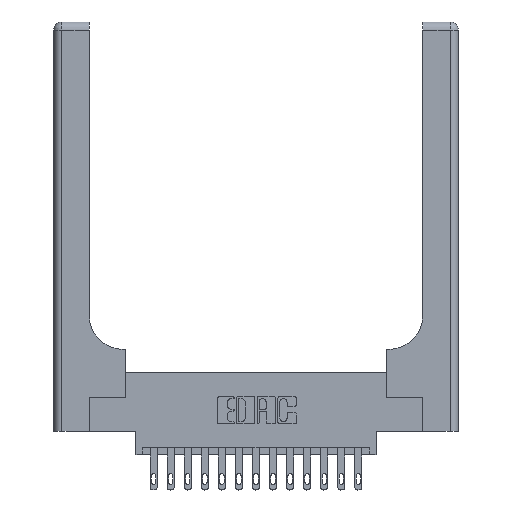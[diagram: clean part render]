
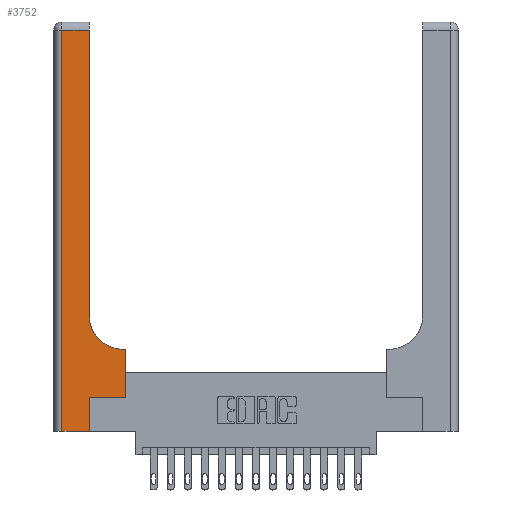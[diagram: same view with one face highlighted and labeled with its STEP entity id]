
A CAD part, top view. The second image highlights one B-rep face of the part: STEP entity #3752.
In plain terms, the highlighted planar face has unit normal (0, 0, 1).
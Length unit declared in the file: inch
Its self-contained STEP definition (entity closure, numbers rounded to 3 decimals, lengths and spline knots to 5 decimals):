
#110 = VECTOR ( 'NONE', #6248, 39.37008 ) ;
#417 = DIRECTION ( 'NONE',  ( -1., 0., 0. ) ) ;
#496 = DIRECTION ( 'NONE',  ( 0., 0., -1. ) ) ;
#1098 = VECTOR ( 'NONE', #417, 39.37008 ) ;
#1609 = VECTOR ( 'NONE', #12902, 39.37008 ) ;
#1746 = CARTESIAN_POINT ( 'NONE',  ( 0.528, 0.25, 0.37 ) ) ;
#1810 = ORIENTED_EDGE ( 'NONE', *, *, #6879, .T. ) ;
#2056 = ORIENTED_EDGE ( 'NONE', *, *, #14182, .T. ) ;
#2074 = DIRECTION ( 'NONE',  ( 1., 0., 0. ) ) ;
#2382 = CARTESIAN_POINT ( 'NONE',  ( 0.26, 2.94, 0.37 ) ) ;
#2437 = ORIENTED_EDGE ( 'NONE', *, *, #6881, .T. ) ;
#2637 = EDGE_CURVE ( 'NONE', #16331, #14171, #12214, .T. ) ;
#3395 = CIRCLE ( 'NONE', #10403, 0.25 ) ;
#3427 = LINE ( 'NONE', #9098, #15426 ) ;
#3638 = DIRECTION ( 'NONE',  ( 0., 0., -1. ) ) ;
#3718 = CARTESIAN_POINT ( 'NONE',  ( 0.06, 2.94, 0.37 ) ) ;
#3752 = ADVANCED_FACE ( 'NONE', ( #4206 ), #14585, .F. ) ;
#4022 = CARTESIAN_POINT ( 'NONE',  ( 0., 0., 0.37 ) ) ;
#4030 = VERTEX_POINT ( 'NONE', #3718 ) ;
#4206 = FACE_OUTER_BOUND ( 'NONE', #14951, .T. ) ;
#5213 = DIRECTION ( 'NONE',  ( -1., 0., 0. ) ) ;
#5225 = VERTEX_POINT ( 'NONE', #11851 ) ;
#5819 = VERTEX_POINT ( 'NONE', #10173 ) ;
#5940 = EDGE_CURVE ( 'NONE', #6156, #16331, #14277, .T. ) ;
#6156 = VERTEX_POINT ( 'NONE', #12410 ) ;
#6248 = DIRECTION ( 'NONE',  ( 0., 1., 0. ) ) ;
#6293 = CARTESIAN_POINT ( 'NONE',  ( 0.51, 0.85, 0.37 ) ) ;
#6533 = DIRECTION ( 'NONE',  ( 0., 1., 0. ) ) ;
#6879 = EDGE_CURVE ( 'NONE', #14171, #17664, #3395, .T. ) ;
#6881 = EDGE_CURVE ( 'NONE', #4030, #5819, #17421, .T. ) ;
#7467 = CARTESIAN_POINT ( 'NONE',  ( 0., 3., 0.37 ) ) ;
#7563 = LINE ( 'NONE', #15866, #1098 ) ;
#7684 = ORIENTED_EDGE ( 'NONE', *, *, #2637, .T. ) ;
#7707 = LINE ( 'NONE', #14547, #110 ) ;
#8044 = EDGE_CURVE ( 'NONE', #5225, #6156, #16064, .T. ) ;
#8217 = LINE ( 'NONE', #4022, #12567 ) ;
#8347 = CARTESIAN_POINT ( 'NONE',  ( 0.26, 0.85, 0.37 ) ) ;
#8474 = CARTESIAN_POINT ( 'NONE',  ( 0.06, 3., 0.37 ) ) ;
#9098 = CARTESIAN_POINT ( 'NONE',  ( 0.265, 0., 0.37 ) ) ;
#9650 = CARTESIAN_POINT ( 'NONE',  ( 0.265, 0., 0.37 ) ) ;
#10173 = CARTESIAN_POINT ( 'NONE',  ( 0.06, 0., 0.37 ) ) ;
#10403 = AXIS2_PLACEMENT_3D ( 'NONE', #6293, #3638, #11833 ) ;
#10613 = ORIENTED_EDGE ( 'NONE', *, *, #10682, .T. ) ;
#10682 = EDGE_CURVE ( 'NONE', #17577, #4030, #7563, .T. ) ;
#10920 = VECTOR ( 'NONE', #5213, 39.37008 ) ;
#11294 = EDGE_CURVE ( 'NONE', #11840, #5225, #3427, .T. ) ;
#11833 = DIRECTION ( 'NONE',  ( 1., 0., 0. ) ) ;
#11840 = VERTEX_POINT ( 'NONE', #9650 ) ;
#11851 = CARTESIAN_POINT ( 'NONE',  ( 0.265, 0.25, 0.37 ) ) ;
#12214 = LINE ( 'NONE', #12388, #10920 ) ;
#12388 = CARTESIAN_POINT ( 'NONE',  ( 0.26, 0.6, 0.37 ) ) ;
#12410 = CARTESIAN_POINT ( 'NONE',  ( 0.528, 0.25, 0.37 ) ) ;
#12567 = VECTOR ( 'NONE', #13595, 39.37008 ) ;
#12706 = ORIENTED_EDGE ( 'NONE', *, *, #11294, .T. ) ;
#12902 = DIRECTION ( 'NONE',  ( 0., 1., 0. ) ) ;
#13026 = DIRECTION ( 'NONE',  ( -1., 0., 0. ) ) ;
#13595 = DIRECTION ( 'NONE',  ( 1., 0., 0. ) ) ;
#13803 = ORIENTED_EDGE ( 'NONE', *, *, #16389, .T. ) ;
#13845 = AXIS2_PLACEMENT_3D ( 'NONE', #7467, #496, #13026 ) ;
#14171 = VERTEX_POINT ( 'NONE', #15796 ) ;
#14182 = EDGE_CURVE ( 'NONE', #5819, #11840, #8217, .T. ) ;
#14277 = LINE ( 'NONE', #1746, #1609 ) ;
#14488 = VECTOR ( 'NONE', #15224, 39.37008 ) ;
#14547 = CARTESIAN_POINT ( 'NONE',  ( 0.26, 3., 0.37 ) ) ;
#14585 = PLANE ( 'NONE',  #13845 ) ;
#14608 = CARTESIAN_POINT ( 'NONE',  ( 0.265, 0.25, 0.37 ) ) ;
#14648 = CARTESIAN_POINT ( 'NONE',  ( 0.528, 0.6, 0.37 ) ) ;
#14951 = EDGE_LOOP ( 'NONE', ( #13803, #10613, #2437, #2056, #12706, #17761, #15083, #7684, #1810 ) ) ;
#15083 = ORIENTED_EDGE ( 'NONE', *, *, #5940, .T. ) ;
#15224 = DIRECTION ( 'NONE',  ( 0., -1., 0. ) ) ;
#15406 = VECTOR ( 'NONE', #2074, 39.37008 ) ;
#15426 = VECTOR ( 'NONE', #6533, 39.37008 ) ;
#15796 = CARTESIAN_POINT ( 'NONE',  ( 0.51, 0.6, 0.37 ) ) ;
#15866 = CARTESIAN_POINT ( 'NONE',  ( 0., 2.94, 0.37 ) ) ;
#16064 = LINE ( 'NONE', #14608, #15406 ) ;
#16331 = VERTEX_POINT ( 'NONE', #14648 ) ;
#16389 = EDGE_CURVE ( 'NONE', #17664, #17577, #7707, .T. ) ;
#17421 = LINE ( 'NONE', #8474, #14488 ) ;
#17577 = VERTEX_POINT ( 'NONE', #2382 ) ;
#17664 = VERTEX_POINT ( 'NONE', #8347 ) ;
#17761 = ORIENTED_EDGE ( 'NONE', *, *, #8044, .T. ) ;
